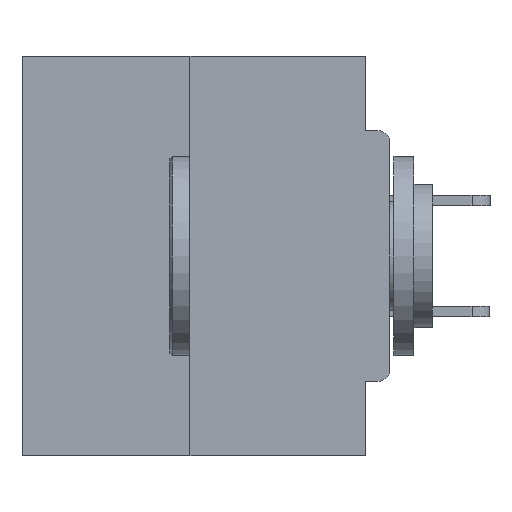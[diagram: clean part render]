
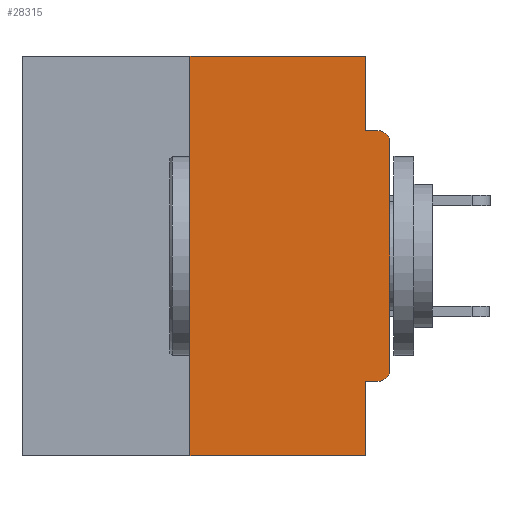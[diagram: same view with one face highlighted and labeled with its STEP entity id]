
A CAD part, left-side view. The second image highlights one B-rep face of the part: STEP entity #28315.
In plain terms, the highlighted planar face has unit normal (-1, 0, 0).
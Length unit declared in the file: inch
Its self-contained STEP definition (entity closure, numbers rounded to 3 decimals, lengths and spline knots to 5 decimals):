
#417 = EDGE_CURVE ( 'NONE', #13257, #16560, #9326, .T. ) ;
#1505 = ORIENTED_EDGE ( 'NONE', *, *, #1696, .F. ) ;
#1696 = EDGE_CURVE ( 'NONE', #10224, #20308, #22827, .T. ) ;
#2373 = CARTESIAN_POINT ( 'NONE',  ( 0., 0.46, -0.5 ) ) ;
#2743 = ORIENTED_EDGE ( 'NONE', *, *, #417, .T. ) ;
#3124 = ORIENTED_EDGE ( 'NONE', *, *, #30465, .T. ) ;
#3320 = EDGE_CURVE ( 'NONE', #27686, #16560, #30521, .T. ) ;
#3474 = CARTESIAN_POINT ( 'NONE',  ( 0., 0., -0.1085 ) ) ;
#4256 = DIRECTION ( 'NONE',  ( 0., 0., -1. ) ) ;
#4403 = PLANE ( 'NONE',  #42688 ) ;
#5260 = CARTESIAN_POINT ( 'NONE',  ( 0., 0.015, -0.4065 ) ) ;
#5718 = VECTOR ( 'NONE', #18478, 39.37008 ) ;
#6448 = CARTESIAN_POINT ( 'NONE',  ( 0., 0.25, 0. ) ) ;
#6678 = ORIENTED_EDGE ( 'NONE', *, *, #13943, .T. ) ;
#6743 = CARTESIAN_POINT ( 'NONE',  ( 0., 0., 0. ) ) ;
#8838 = DIRECTION ( 'NONE',  ( 0., -1., 0. ) ) ;
#9326 = LINE ( 'NONE', #2373, #14042 ) ;
#9759 = EDGE_CURVE ( 'NONE', #20308, #23653, #40380, .T. ) ;
#9857 = CARTESIAN_POINT ( 'NONE',  ( 0., 0.031, -0.4065 ) ) ;
#10224 = VERTEX_POINT ( 'NONE', #13760 ) ;
#11119 = ORIENTED_EDGE ( 'NONE', *, *, #3320, .F. ) ;
#12523 = CARTESIAN_POINT ( 'NONE',  ( 0., 0., -0.4065 ) ) ;
#12730 = CARTESIAN_POINT ( 'NONE',  ( 0., 0.015, -0.0935 ) ) ;
#13257 = VERTEX_POINT ( 'NONE', #33634 ) ;
#13728 = EDGE_CURVE ( 'NONE', #18397, #10224, #16694, .T. ) ;
#13760 = CARTESIAN_POINT ( 'NONE',  ( 0., 0.031, 0. ) ) ;
#13943 = EDGE_CURVE ( 'NONE', #33969, #40918, #16162, .T. ) ;
#14042 = VECTOR ( 'NONE', #8838, 39.37008 ) ;
#14244 = DIRECTION ( 'NONE',  ( 1., 0., 0. ) ) ;
#14587 = VECTOR ( 'NONE', #40932, 39.37008 ) ;
#14872 = FACE_OUTER_BOUND ( 'NONE', #15472, .T. ) ;
#15472 = EDGE_LOOP ( 'NONE', ( #34892, #20325, #2743, #11119, #18050, #6678, #3124, #20740, #23274, #1505 ) ) ;
#16162 = CIRCLE ( 'NONE', #37104, 0.015 ) ;
#16560 = VERTEX_POINT ( 'NONE', #36773 ) ;
#16694 = LINE ( 'NONE', #39651, #26176 ) ;
#17074 = CARTESIAN_POINT ( 'NONE',  ( 0., 0.015, -0.3915 ) ) ;
#17197 = VECTOR ( 'NONE', #26656, 39.37008 ) ;
#18050 = ORIENTED_EDGE ( 'NONE', *, *, #32598, .F. ) ;
#18379 = VECTOR ( 'NONE', #41080, 39.37008 ) ;
#18397 = VERTEX_POINT ( 'NONE', #6448 ) ;
#18478 = DIRECTION ( 'NONE',  ( 0., 1., 0. ) ) ;
#19349 = LINE ( 'NONE', #12523, #5718 ) ;
#20308 = VERTEX_POINT ( 'NONE', #24384 ) ;
#20325 = ORIENTED_EDGE ( 'NONE', *, *, #25931, .F. ) ;
#20740 = ORIENTED_EDGE ( 'NONE', *, *, #20757, .T. ) ;
#20757 = EDGE_CURVE ( 'NONE', #24959, #23653, #39337, .T. ) ;
#21790 = DIRECTION ( 'NONE',  ( 0., 0., -1. ) ) ;
#21938 = CARTESIAN_POINT ( 'NONE',  ( 0., 0.015, -0.1085 ) ) ;
#22827 = LINE ( 'NONE', #22868, #29649 ) ;
#22868 = CARTESIAN_POINT ( 'NONE',  ( 0., 0.031, 0. ) ) ;
#23274 = ORIENTED_EDGE ( 'NONE', *, *, #9759, .F. ) ;
#23653 = VERTEX_POINT ( 'NONE', #12730 ) ;
#24384 = CARTESIAN_POINT ( 'NONE',  ( 0., 0.031, -0.0935 ) ) ;
#24959 = VERTEX_POINT ( 'NONE', #3474 ) ;
#25931 = EDGE_CURVE ( 'NONE', #13257, #18397, #37254, .T. ) ;
#26176 = VECTOR ( 'NONE', #42861, 39.37008 ) ;
#26392 = DIRECTION ( 'NONE',  ( 0., 0., 1. ) ) ;
#26656 = DIRECTION ( 'NONE',  ( 0., 0., 1. ) ) ;
#27686 = VERTEX_POINT ( 'NONE', #9857 ) ;
#28098 = CARTESIAN_POINT ( 'NONE',  ( 0., 0.031, -0.5 ) ) ;
#28315 = ADVANCED_FACE ( 'NONE', ( #14872 ), #4403, .F. ) ;
#29023 = DIRECTION ( 'NONE',  ( 0., 0., -1. ) ) ;
#29649 = VECTOR ( 'NONE', #29023, 39.37008 ) ;
#30465 = EDGE_CURVE ( 'NONE', #40918, #24959, #43106, .T. ) ;
#30521 = LINE ( 'NONE', #28098, #18379 ) ;
#30747 = CARTESIAN_POINT ( 'NONE',  ( 0., 0., -0.0935 ) ) ;
#32598 = EDGE_CURVE ( 'NONE', #33969, #27686, #19349, .T. ) ;
#33634 = CARTESIAN_POINT ( 'NONE',  ( 0., 0.25, -0.5 ) ) ;
#33969 = VERTEX_POINT ( 'NONE', #5260 ) ;
#34112 = CARTESIAN_POINT ( 'NONE',  ( 0., 0.46, 0. ) ) ;
#34892 = ORIENTED_EDGE ( 'NONE', *, *, #13728, .F. ) ;
#35773 = VECTOR ( 'NONE', #26392, 39.37008 ) ;
#36773 = CARTESIAN_POINT ( 'NONE',  ( 0., 0.031, -0.5 ) ) ;
#37104 = AXIS2_PLACEMENT_3D ( 'NONE', #17074, #40796, #41068 ) ;
#37254 = LINE ( 'NONE', #40231, #17197 ) ;
#39337 = CIRCLE ( 'NONE', #41660, 0.015 ) ;
#39475 = CARTESIAN_POINT ( 'NONE',  ( 0., 0., -0.3915 ) ) ;
#39651 = CARTESIAN_POINT ( 'NONE',  ( 0., 0.46, 0. ) ) ;
#40231 = CARTESIAN_POINT ( 'NONE',  ( 0., 0.25, 0. ) ) ;
#40380 = LINE ( 'NONE', #30747, #14587 ) ;
#40796 = DIRECTION ( 'NONE',  ( -1., 0., 0. ) ) ;
#40918 = VERTEX_POINT ( 'NONE', #39475 ) ;
#40932 = DIRECTION ( 'NONE',  ( 0., -1., 0. ) ) ;
#41068 = DIRECTION ( 'NONE',  ( 0., 0., -1. ) ) ;
#41080 = DIRECTION ( 'NONE',  ( 0., 0., -1. ) ) ;
#41501 = DIRECTION ( 'NONE',  ( -1., 0., 0. ) ) ;
#41660 = AXIS2_PLACEMENT_3D ( 'NONE', #21938, #41501, #21790 ) ;
#42688 = AXIS2_PLACEMENT_3D ( 'NONE', #34112, #14244, #4256 ) ;
#42861 = DIRECTION ( 'NONE',  ( 0., -1., 0. ) ) ;
#43106 = LINE ( 'NONE', #6743, #35773 ) ;
